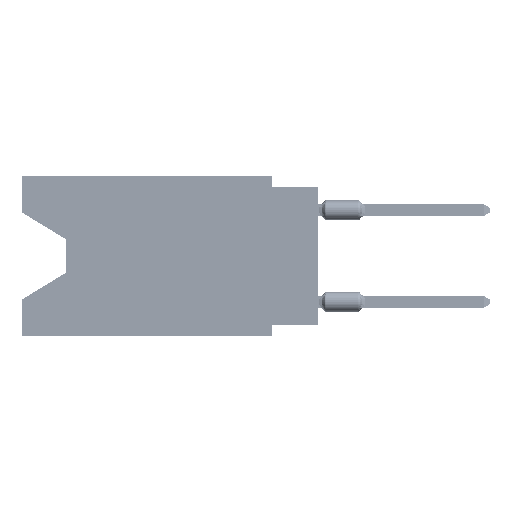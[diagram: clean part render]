
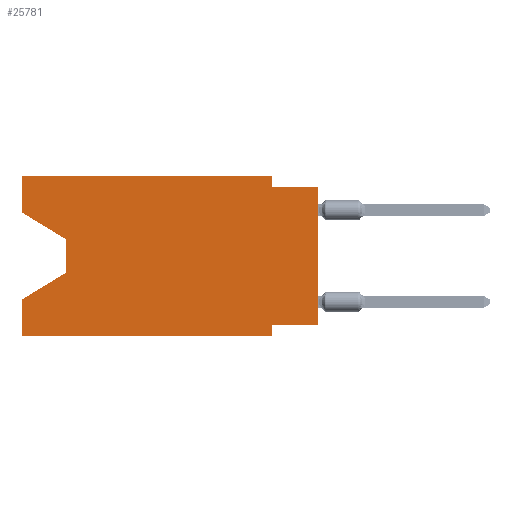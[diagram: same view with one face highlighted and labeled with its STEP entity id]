
A CAD part, left-side view. The second image highlights one B-rep face of the part: STEP entity #25781.
In plain terms, the highlighted planar face has unit normal (-1, 0, 0).
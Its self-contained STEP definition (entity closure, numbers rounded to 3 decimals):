
#391 = EDGE_CURVE ( 'NONE', #41614, #93474, #2387, .T. ) ;
#1548 = CARTESIAN_POINT ( 'NONE',  ( 0., 2.54, -8.89 ) ) ;
#1942 = ORIENTED_EDGE ( 'NONE', *, *, #17613, .F. ) ;
#2387 = LINE ( 'NONE', #32777, #59878 ) ;
#2651 = LINE ( 'NONE', #18325, #88534 ) ;
#3135 = DIRECTION ( 'NONE',  ( 0., 0., 1. ) ) ;
#3505 = ORIENTED_EDGE ( 'NONE', *, *, #16298, .F. ) ;
#3927 = DIRECTION ( 'NONE',  ( 0., 0., 1. ) ) ;
#7530 = VECTOR ( 'NONE', #3927, 1000. ) ;
#8821 = LINE ( 'NONE', #80115, #38455 ) ;
#9614 = CARTESIAN_POINT ( 'NONE',  ( 0., 0., 0. ) ) ;
#10577 = LINE ( 'NONE', #9614, #56888 ) ;
#11841 = CARTESIAN_POINT ( 'NONE',  ( 0., 0., -8.255 ) ) ;
#14934 = DIRECTION ( 'NONE',  ( 0., 0.855, -0.519 ) ) ;
#15527 = CARTESIAN_POINT ( 'NONE',  ( 0., 16.383, 0. ) ) ;
#16011 = ORIENTED_EDGE ( 'NONE', *, *, #35217, .T. ) ;
#16298 = EDGE_CURVE ( 'NONE', #48443, #64734, #2651, .T. ) ;
#17578 = LINE ( 'NONE', #71961, #46120 ) ;
#17613 = EDGE_CURVE ( 'NONE', #46859, #93474, #40691, .T. ) ;
#18325 = CARTESIAN_POINT ( 'NONE',  ( 0., 16.383, 0. ) ) ;
#20162 = EDGE_CURVE ( 'NONE', #64734, #42173, #58773, .T. ) ;
#20576 = ORIENTED_EDGE ( 'NONE', *, *, #71696, .F. ) ;
#20706 = ORIENTED_EDGE ( 'NONE', *, *, #40376, .F. ) ;
#21245 = VECTOR ( 'NONE', #45678, 1000. ) ;
#22520 = VERTEX_POINT ( 'NONE', #91815 ) ;
#23811 = CARTESIAN_POINT ( 'NONE',  ( 0., 0., -8.255 ) ) ;
#24053 = DIRECTION ( 'NONE',  ( 0., -1., 0. ) ) ;
#24086 = DIRECTION ( 'NONE',  ( 0., 0., -1. ) ) ;
#24695 = VECTOR ( 'NONE', #33554, 1000. ) ;
#25175 = DIRECTION ( 'NONE',  ( 0., -1., 0. ) ) ;
#25781 = ADVANCED_FACE ( 'NONE', ( #85965 ), #63184, .F. ) ;
#26593 = CARTESIAN_POINT ( 'NONE',  ( 0., 16.383, 0. ) ) ;
#27969 = CARTESIAN_POINT ( 'NONE',  ( 0., 16.383, 0. ) ) ;
#28481 = DIRECTION ( 'NONE',  ( 1., 0., 0. ) ) ;
#29306 = VERTEX_POINT ( 'NONE', #34808 ) ;
#31214 = CARTESIAN_POINT ( 'NONE',  ( 0., 16.383, -2.038 ) ) ;
#32765 = CARTESIAN_POINT ( 'NONE',  ( 0., 16.383, -2.038 ) ) ;
#32777 = CARTESIAN_POINT ( 'NONE',  ( 0., 16.383, -8.89 ) ) ;
#33409 = CARTESIAN_POINT ( 'NONE',  ( 0., 16.383, 0. ) ) ;
#33554 = DIRECTION ( 'NONE',  ( 0., 0., -1. ) ) ;
#34808 = CARTESIAN_POINT ( 'NONE',  ( 0., 13.97, -3.505 ) ) ;
#34832 = CARTESIAN_POINT ( 'NONE',  ( 0., 16.383, -8.89 ) ) ;
#35217 = EDGE_CURVE ( 'NONE', #50038, #91220, #10577, .T. ) ;
#38455 = VECTOR ( 'NONE', #44453, 1000. ) ;
#39491 = LINE ( 'NONE', #23811, #21245 ) ;
#40376 = EDGE_CURVE ( 'NONE', #41614, #22520, #85166, .T. ) ;
#40691 = LINE ( 'NONE', #84374, #24695 ) ;
#41508 = ORIENTED_EDGE ( 'NONE', *, *, #42541, .F. ) ;
#41614 = VERTEX_POINT ( 'NONE', #34832 ) ;
#42173 = VERTEX_POINT ( 'NONE', #74159 ) ;
#42541 = EDGE_CURVE ( 'NONE', #50629, #91220, #73569, .T. ) ;
#43380 = ORIENTED_EDGE ( 'NONE', *, *, #63192, .F. ) ;
#44453 = DIRECTION ( 'NONE',  ( 0., 0., -1. ) ) ;
#45678 = DIRECTION ( 'NONE',  ( 0., 1., 0. ) ) ;
#45927 = CARTESIAN_POINT ( 'NONE',  ( 0., 2.54, 0. ) ) ;
#46120 = VECTOR ( 'NONE', #14934, 1000. ) ;
#46275 = CARTESIAN_POINT ( 'NONE',  ( 0., 13.97, -5.385 ) ) ;
#46332 = VECTOR ( 'NONE', #24053, 1000. ) ;
#46859 = VERTEX_POINT ( 'NONE', #78474 ) ;
#48443 = VERTEX_POINT ( 'NONE', #32765 ) ;
#49518 = EDGE_CURVE ( 'NONE', #67269, #22520, #17578, .T. ) ;
#49702 = EDGE_CURVE ( 'NONE', #48443, #29306, #90121, .T. ) ;
#50038 = VERTEX_POINT ( 'NONE', #11841 ) ;
#50629 = VERTEX_POINT ( 'NONE', #85802 ) ;
#50749 = ORIENTED_EDGE ( 'NONE', *, *, #49702, .T. ) ;
#55253 = ORIENTED_EDGE ( 'NONE', *, *, #60910, .T. ) ;
#56888 = VECTOR ( 'NONE', #61387, 1000. ) ;
#57702 = VECTOR ( 'NONE', #89210, 1000. ) ;
#58326 = AXIS2_PLACEMENT_3D ( 'NONE', #26593, #28481, #93097 ) ;
#58773 = LINE ( 'NONE', #15527, #46332 ) ;
#59731 = DIRECTION ( 'NONE',  ( 0., -0.855, -0.519 ) ) ;
#59878 = VECTOR ( 'NONE', #25175, 1000. ) ;
#60910 = EDGE_CURVE ( 'NONE', #29306, #67269, #8821, .T. ) ;
#61012 = ORIENTED_EDGE ( 'NONE', *, *, #391, .T. ) ;
#61387 = DIRECTION ( 'NONE',  ( 0., 0., 1. ) ) ;
#63184 = PLANE ( 'NONE',  #58326 ) ;
#63192 = EDGE_CURVE ( 'NONE', #42173, #50629, #88702, .T. ) ;
#64734 = VERTEX_POINT ( 'NONE', #27969 ) ;
#65879 = VECTOR ( 'NONE', #59731, 1000. ) ;
#66903 = CARTESIAN_POINT ( 'NONE',  ( 0., 0., -0.635 ) ) ;
#67269 = VERTEX_POINT ( 'NONE', #46275 ) ;
#68362 = EDGE_LOOP ( 'NONE', ( #50749, #55253, #90573, #20706, #61012, #1942, #20576, #16011, #41508, #43380, #81747, #3505 ) ) ;
#69817 = CARTESIAN_POINT ( 'NONE',  ( 0., 0., -0.635 ) ) ;
#71696 = EDGE_CURVE ( 'NONE', #50038, #46859, #39491, .T. ) ;
#71961 = CARTESIAN_POINT ( 'NONE',  ( 0., 13.97, -5.385 ) ) ;
#73485 = VECTOR ( 'NONE', #24086, 1000. ) ;
#73569 = LINE ( 'NONE', #66903, #57702 ) ;
#74159 = CARTESIAN_POINT ( 'NONE',  ( 0., 2.54, 0. ) ) ;
#78474 = CARTESIAN_POINT ( 'NONE',  ( 0., 2.54, -8.255 ) ) ;
#80115 = CARTESIAN_POINT ( 'NONE',  ( 0., 13.97, -3.505 ) ) ;
#81747 = ORIENTED_EDGE ( 'NONE', *, *, #20162, .F. ) ;
#84374 = CARTESIAN_POINT ( 'NONE',  ( 0., 2.54, -8.89 ) ) ;
#85166 = LINE ( 'NONE', #33409, #7530 ) ;
#85802 = CARTESIAN_POINT ( 'NONE',  ( 0., 2.54, -0.635 ) ) ;
#85965 = FACE_OUTER_BOUND ( 'NONE', #68362, .T. ) ;
#88534 = VECTOR ( 'NONE', #3135, 1000. ) ;
#88702 = LINE ( 'NONE', #45927, #73485 ) ;
#89210 = DIRECTION ( 'NONE',  ( 0., -1., 0. ) ) ;
#90121 = LINE ( 'NONE', #31214, #65879 ) ;
#90573 = ORIENTED_EDGE ( 'NONE', *, *, #49518, .T. ) ;
#91220 = VERTEX_POINT ( 'NONE', #69817 ) ;
#91815 = CARTESIAN_POINT ( 'NONE',  ( 0., 16.383, -6.852 ) ) ;
#93097 = DIRECTION ( 'NONE',  ( 0., 0., -1. ) ) ;
#93474 = VERTEX_POINT ( 'NONE', #1548 ) ;
